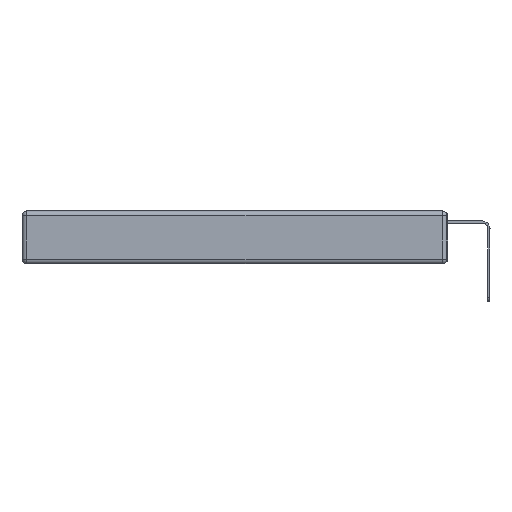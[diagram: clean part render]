
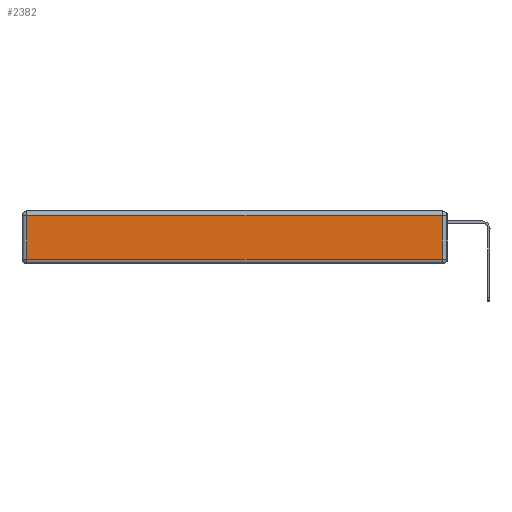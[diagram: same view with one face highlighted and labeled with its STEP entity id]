
A CAD part, left-side view. The second image highlights one B-rep face of the part: STEP entity #2382.
In plain terms, the highlighted planar face has unit normal (-1, 0, 0).
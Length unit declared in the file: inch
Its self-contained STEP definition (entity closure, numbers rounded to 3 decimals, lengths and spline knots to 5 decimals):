
#1696 = DIRECTION ( 'NONE',  ( 0., 0., 1. ) ) ;
#2382 = ADVANCED_FACE ( 'NONE', ( #7796 ), #11663, .T. ) ;
#2625 = CARTESIAN_POINT ( 'NONE',  ( 0., 2.75, -0.03 ) ) ;
#2686 = DIRECTION ( 'NONE',  ( 0., -1., 0. ) ) ;
#4410 = EDGE_CURVE ( 'NONE', #13755, #22831, #13691, .T. ) ;
#7796 = FACE_OUTER_BOUND ( 'NONE', #8598, .T. ) ;
#7803 = LINE ( 'NONE', #2625, #23616 ) ;
#8479 = CARTESIAN_POINT ( 'NONE',  ( 0., 2.72, -0.03 ) ) ;
#8598 = EDGE_LOOP ( 'NONE', ( #22152, #24434, #24768, #21100 ) ) ;
#8618 = DIRECTION ( 'NONE',  ( 0., 1., 0. ) ) ;
#8686 = CARTESIAN_POINT ( 'NONE',  ( 0., 0., -0.313 ) ) ;
#9780 = LINE ( 'NONE', #23503, #21547 ) ;
#11663 = PLANE ( 'NONE',  #19913 ) ;
#12560 = EDGE_CURVE ( 'NONE', #22831, #24763, #20359, .T. ) ;
#13691 = LINE ( 'NONE', #8686, #22046 ) ;
#13755 = VERTEX_POINT ( 'NONE', #16992 ) ;
#15553 = DIRECTION ( 'NONE',  ( 0., 0., -1. ) ) ;
#16544 = CARTESIAN_POINT ( 'NONE',  ( 0., 0.03, -0.343 ) ) ;
#16992 = CARTESIAN_POINT ( 'NONE',  ( 0., 2.72, -0.313 ) ) ;
#17449 = DIRECTION ( 'NONE',  ( -1., 0., 0. ) ) ;
#18333 = CARTESIAN_POINT ( 'NONE',  ( 0., 0.03, -0.313 ) ) ;
#18481 = VERTEX_POINT ( 'NONE', #8479 ) ;
#19412 = VECTOR ( 'NONE', #24519, 39.37008 ) ;
#19559 = EDGE_CURVE ( 'NONE', #18481, #13755, #9780, .T. ) ;
#19913 = AXIS2_PLACEMENT_3D ( 'NONE', #21360, #17449, #1696 ) ;
#20359 = LINE ( 'NONE', #16544, #19412 ) ;
#21100 = ORIENTED_EDGE ( 'NONE', *, *, #19559, .T. ) ;
#21360 = CARTESIAN_POINT ( 'NONE',  ( 0., 0., -0.343 ) ) ;
#21547 = VECTOR ( 'NONE', #15553, 39.37008 ) ;
#22046 = VECTOR ( 'NONE', #2686, 39.37008 ) ;
#22152 = ORIENTED_EDGE ( 'NONE', *, *, #4410, .T. ) ;
#22428 = CARTESIAN_POINT ( 'NONE',  ( 0., 0.03, -0.03 ) ) ;
#22548 = EDGE_CURVE ( 'NONE', #24763, #18481, #7803, .T. ) ;
#22831 = VERTEX_POINT ( 'NONE', #18333 ) ;
#23503 = CARTESIAN_POINT ( 'NONE',  ( 0., 2.72, -0.343 ) ) ;
#23616 = VECTOR ( 'NONE', #8618, 39.37008 ) ;
#24434 = ORIENTED_EDGE ( 'NONE', *, *, #12560, .T. ) ;
#24519 = DIRECTION ( 'NONE',  ( 0., 0., 1. ) ) ;
#24763 = VERTEX_POINT ( 'NONE', #22428 ) ;
#24768 = ORIENTED_EDGE ( 'NONE', *, *, #22548, .T. ) ;
